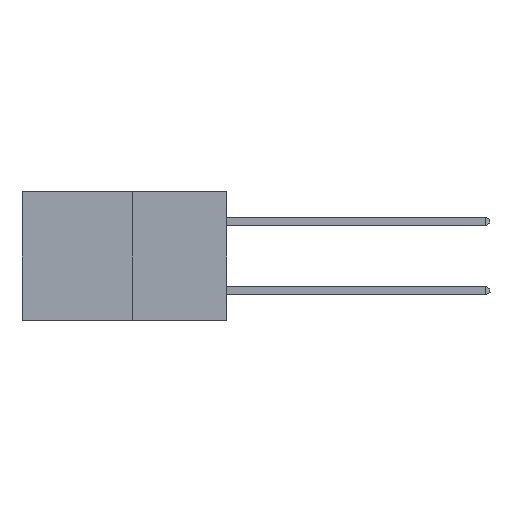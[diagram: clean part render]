
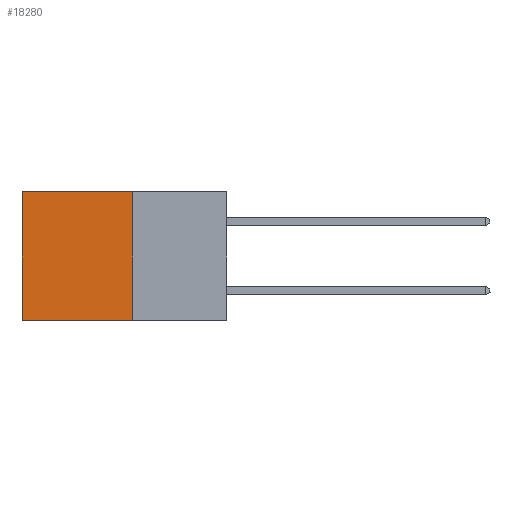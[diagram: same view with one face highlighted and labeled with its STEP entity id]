
A CAD part, left-side view. The second image highlights one B-rep face of the part: STEP entity #18280.
In plain terms, the highlighted planar face has unit normal (-1, 0, 0).
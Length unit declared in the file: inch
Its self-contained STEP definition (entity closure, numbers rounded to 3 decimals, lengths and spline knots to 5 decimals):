
#718 = VECTOR ( 'NONE', #8357, 39.37008 ) ;
#1485 = CARTESIAN_POINT ( 'NONE',  ( 0.277, 0.59, 0. ) ) ;
#1902 = VECTOR ( 'NONE', #14380, 39.37008 ) ;
#2503 = LINE ( 'NONE', #2811, #718 ) ;
#2811 = CARTESIAN_POINT ( 'NONE',  ( 0.277, 0.27, -0.37 ) ) ;
#3222 = CARTESIAN_POINT ( 'NONE',  ( 0.277, 0.27, -0.37 ) ) ;
#4229 = FACE_OUTER_BOUND ( 'NONE', #8829, .T. ) ;
#4760 = PLANE ( 'NONE',  #36017 ) ;
#4807 = VERTEX_POINT ( 'NONE', #21459 ) ;
#7729 = DIRECTION ( 'NONE',  ( 0., 0., -1. ) ) ;
#8357 = DIRECTION ( 'NONE',  ( 0., 0., -1. ) ) ;
#8829 = EDGE_LOOP ( 'NONE', ( #9723, #24971, #25292, #24024 ) ) ;
#8876 = DIRECTION ( 'NONE',  ( 0., 1., 0. ) ) ;
#9723 = ORIENTED_EDGE ( 'NONE', *, *, #11925, .T. ) ;
#10511 = EDGE_CURVE ( 'NONE', #19763, #4807, #23751, .T. ) ;
#11925 = EDGE_CURVE ( 'NONE', #30900, #4807, #14101, .T. ) ;
#14101 = LINE ( 'NONE', #17012, #28180 ) ;
#14189 = DIRECTION ( 'NONE',  ( 0., 0., -1. ) ) ;
#14380 = DIRECTION ( 'NONE',  ( 0., 1., 0. ) ) ;
#16101 = CARTESIAN_POINT ( 'NONE',  ( 0.277, 0.27, -0.37 ) ) ;
#16305 = VECTOR ( 'NONE', #8876, 39.37008 ) ;
#16898 = LINE ( 'NONE', #22742, #1902 ) ;
#17012 = CARTESIAN_POINT ( 'NONE',  ( 0.277, 0.59, -0.37 ) ) ;
#17915 = EDGE_CURVE ( 'NONE', #33252, #19763, #2503, .T. ) ;
#18280 = ADVANCED_FACE ( 'NONE', ( #4229 ), #4760, .F. ) ;
#19763 = VERTEX_POINT ( 'NONE', #33084 ) ;
#19986 = EDGE_CURVE ( 'NONE', #33252, #30900, #16898, .T. ) ;
#21459 = CARTESIAN_POINT ( 'NONE',  ( 0.277, 0.59, -0.37 ) ) ;
#22742 = CARTESIAN_POINT ( 'NONE',  ( 0.277, 0.27, 0. ) ) ;
#23751 = LINE ( 'NONE', #3222, #16305 ) ;
#24024 = ORIENTED_EDGE ( 'NONE', *, *, #19986, .T. ) ;
#24570 = DIRECTION ( 'NONE',  ( 1., 0., 0. ) ) ;
#24971 = ORIENTED_EDGE ( 'NONE', *, *, #10511, .F. ) ;
#25292 = ORIENTED_EDGE ( 'NONE', *, *, #17915, .F. ) ;
#28180 = VECTOR ( 'NONE', #14189, 39.37008 ) ;
#30900 = VERTEX_POINT ( 'NONE', #1485 ) ;
#31006 = CARTESIAN_POINT ( 'NONE',  ( 0.277, 0.27, 0. ) ) ;
#33084 = CARTESIAN_POINT ( 'NONE',  ( 0.277, 0.27, -0.37 ) ) ;
#33252 = VERTEX_POINT ( 'NONE', #31006 ) ;
#36017 = AXIS2_PLACEMENT_3D ( 'NONE', #16101, #24570, #7729 ) ;
